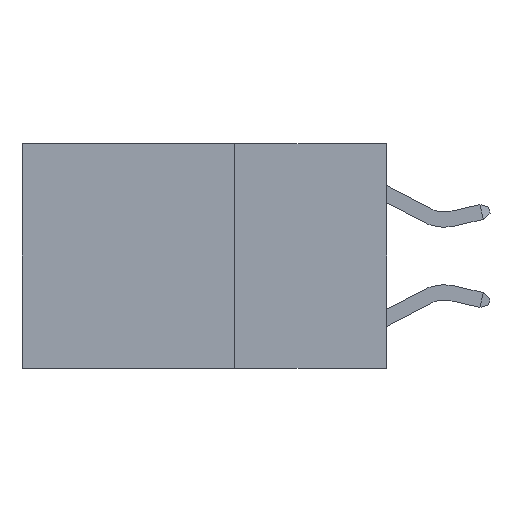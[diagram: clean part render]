
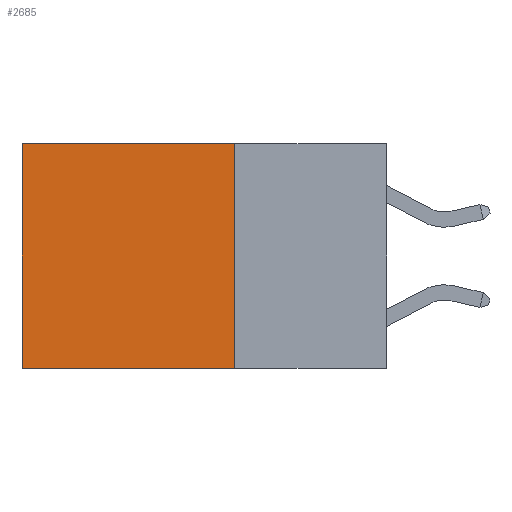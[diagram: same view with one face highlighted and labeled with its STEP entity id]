
A CAD part, left-side view. The second image highlights one B-rep face of the part: STEP entity #2685.
In plain terms, the highlighted planar face has unit normal (-1, 0, 0).
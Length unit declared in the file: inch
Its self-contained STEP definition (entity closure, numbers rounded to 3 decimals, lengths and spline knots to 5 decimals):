
#44 = EDGE_CURVE ( 'NONE', #805, #5655, #7200, .T. ) ;
#104 = PLANE ( 'NONE',  #5948 ) ;
#805 = VERTEX_POINT ( 'NONE', #5142 ) ;
#883 = DIRECTION ( 'NONE',  ( 0., 0., -1. ) ) ;
#973 = CARTESIAN_POINT ( 'NONE',  ( 0.2625, 0.25, 0. ) ) ;
#1067 = LINE ( 'NONE', #1475, #8582 ) ;
#1475 = CARTESIAN_POINT ( 'NONE',  ( 0.2625, 0.25, -0.37 ) ) ;
#1776 = DIRECTION ( 'NONE',  ( 0., 1., 0. ) ) ;
#1895 = FACE_OUTER_BOUND ( 'NONE', #6987, .T. ) ;
#2049 = LINE ( 'NONE', #2962, #3914 ) ;
#2416 = CARTESIAN_POINT ( 'NONE',  ( 0.2625, 0.25, 0. ) ) ;
#2685 = ADVANCED_FACE ( 'NONE', ( #1895 ), #104, .F. ) ;
#2962 = CARTESIAN_POINT ( 'NONE',  ( 0.2625, 0.6, 0. ) ) ;
#3334 = VECTOR ( 'NONE', #7872, 39.37008 ) ;
#3914 = VECTOR ( 'NONE', #8639, 39.37008 ) ;
#4050 = EDGE_CURVE ( 'NONE', #805, #4992, #6499, .T. ) ;
#4831 = EDGE_CURVE ( 'NONE', #4992, #8538, #2049, .T. ) ;
#4992 = VERTEX_POINT ( 'NONE', #8154 ) ;
#5142 = CARTESIAN_POINT ( 'NONE',  ( 0.2625, 0.25, 0. ) ) ;
#5438 = DIRECTION ( 'NONE',  ( 1., 0., 0. ) ) ;
#5655 = VERTEX_POINT ( 'NONE', #7418 ) ;
#5657 = EDGE_CURVE ( 'NONE', #5655, #8538, #1067, .T. ) ;
#5948 = AXIS2_PLACEMENT_3D ( 'NONE', #2416, #5438, #883 ) ;
#6294 = VECTOR ( 'NONE', #1776, 39.37008 ) ;
#6499 = LINE ( 'NONE', #973, #6294 ) ;
#6683 = CARTESIAN_POINT ( 'NONE',  ( 0.2625, 0.25, 0. ) ) ;
#6987 = EDGE_LOOP ( 'NONE', ( #8738, #8750, #8770, #8776 ) ) ;
#7200 = LINE ( 'NONE', #6683, #3334 ) ;
#7418 = CARTESIAN_POINT ( 'NONE',  ( 0.2625, 0.25, -0.37 ) ) ;
#7443 = DIRECTION ( 'NONE',  ( 0., 1., 0. ) ) ;
#7461 = CARTESIAN_POINT ( 'NONE',  ( 0.2625, 0.6, -0.37 ) ) ;
#7872 = DIRECTION ( 'NONE',  ( 0., 0., -1. ) ) ;
#8154 = CARTESIAN_POINT ( 'NONE',  ( 0.2625, 0.6, 0. ) ) ;
#8538 = VERTEX_POINT ( 'NONE', #7461 ) ;
#8582 = VECTOR ( 'NONE', #7443, 39.37008 ) ;
#8639 = DIRECTION ( 'NONE',  ( 0., 0., -1. ) ) ;
#8738 = ORIENTED_EDGE ( 'NONE', *, *, #4831, .T. ) ;
#8750 = ORIENTED_EDGE ( 'NONE', *, *, #5657, .F. ) ;
#8770 = ORIENTED_EDGE ( 'NONE', *, *, #44, .F. ) ;
#8776 = ORIENTED_EDGE ( 'NONE', *, *, #4050, .T. ) ;
